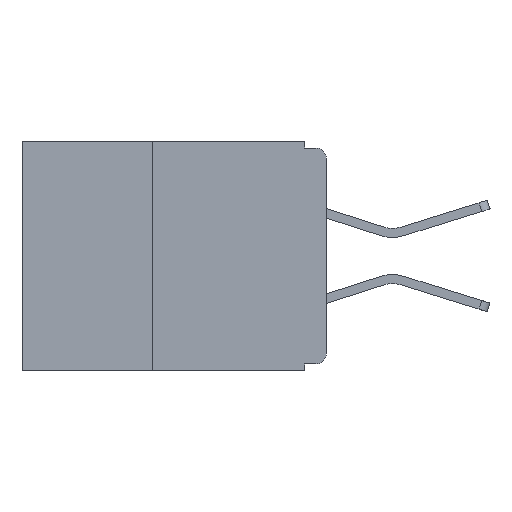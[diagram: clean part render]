
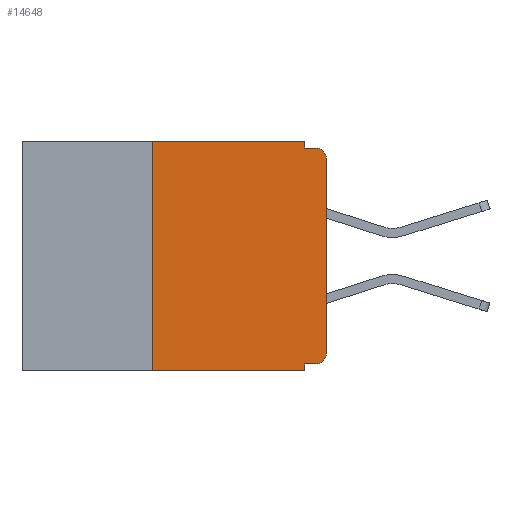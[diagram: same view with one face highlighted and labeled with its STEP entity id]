
A CAD part, left-side view. The second image highlights one B-rep face of the part: STEP entity #14648.
In plain terms, the highlighted planar face has unit normal (-1, 0, 0).
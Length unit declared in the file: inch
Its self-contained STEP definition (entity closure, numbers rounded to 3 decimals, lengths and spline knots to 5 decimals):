
#143 = LINE ( 'NONE', #12349, #18128 ) ;
#157 = VERTEX_POINT ( 'NONE', #21120 ) ;
#232 = DIRECTION ( 'NONE',  ( 0., 0., -1. ) ) ;
#410 = DIRECTION ( 'NONE',  ( 0., 0., -1. ) ) ;
#474 = DIRECTION ( 'NONE',  ( 0., -1., 0. ) ) ;
#589 = PLANE ( 'NONE',  #3066 ) ;
#1027 = LINE ( 'NONE', #11122, #20057 ) ;
#1802 = EDGE_CURVE ( 'NONE', #10880, #9495, #7541, .T. ) ;
#1854 = CARTESIAN_POINT ( 'NONE',  ( 0., 0.437, -0.33 ) ) ;
#2018 = VECTOR ( 'NONE', #2276, 39.37008 ) ;
#2039 = FACE_OUTER_BOUND ( 'NONE', #3339, .T. ) ;
#2276 = DIRECTION ( 'NONE',  ( 0., -1., 0. ) ) ;
#2361 = VECTOR ( 'NONE', #410, 39.37008 ) ;
#2442 = DIRECTION ( 'NONE',  ( 1., 0., 0. ) ) ;
#2985 = LINE ( 'NONE', #9601, #12583 ) ;
#3066 = AXIS2_PLACEMENT_3D ( 'NONE', #13242, #2442, #15018 ) ;
#3339 = EDGE_LOOP ( 'NONE', ( #22673, #15878, #10352, #20879, #21945, #16506, #5293, #3642, #5129, #12733 ) ) ;
#3525 = VECTOR ( 'NONE', #16379, 39.37008 ) ;
#3642 = ORIENTED_EDGE ( 'NONE', *, *, #8073, .F. ) ;
#4120 = CARTESIAN_POINT ( 'NONE',  ( 0., 0.437, 0. ) ) ;
#5129 = ORIENTED_EDGE ( 'NONE', *, *, #21127, .F. ) ;
#5293 = ORIENTED_EDGE ( 'NONE', *, *, #1802, .T. ) ;
#5303 = EDGE_CURVE ( 'NONE', #10880, #18103, #143, .T. ) ;
#6342 = CARTESIAN_POINT ( 'NONE',  ( 0., 0., 0. ) ) ;
#7115 = CARTESIAN_POINT ( 'NONE',  ( 0., 0.25, 0. ) ) ;
#7248 = AXIS2_PLACEMENT_3D ( 'NONE', #18072, #7424, #19826 ) ;
#7424 = DIRECTION ( 'NONE',  ( -1., 0., 0. ) ) ;
#7541 = LINE ( 'NONE', #1854, #11209 ) ;
#7942 = VERTEX_POINT ( 'NONE', #9191 ) ;
#8073 = EDGE_CURVE ( 'NONE', #7942, #9495, #21308, .T. ) ;
#9191 = CARTESIAN_POINT ( 'NONE',  ( 0., 0.031, -0.32 ) ) ;
#9495 = VERTEX_POINT ( 'NONE', #17965 ) ;
#9601 = CARTESIAN_POINT ( 'NONE',  ( 0., 0., -0.01 ) ) ;
#9658 = CARTESIAN_POINT ( 'NONE',  ( 0., 0.015, -0.01 ) ) ;
#9702 = CARTESIAN_POINT ( 'NONE',  ( 0., 0.015, -0.025 ) ) ;
#10116 = CIRCLE ( 'NONE', #7248, 0.015 ) ;
#10352 = ORIENTED_EDGE ( 'NONE', *, *, #22481, .F. ) ;
#10839 = EDGE_CURVE ( 'NONE', #19316, #157, #1027, .T. ) ;
#10851 = CARTESIAN_POINT ( 'NONE',  ( 0., 0.015, -0.32 ) ) ;
#10880 = VERTEX_POINT ( 'NONE', #14759 ) ;
#10893 = CARTESIAN_POINT ( 'NONE',  ( 0., 0., -0.305 ) ) ;
#11117 = EDGE_CURVE ( 'NONE', #19611, #15234, #19220, .T. ) ;
#11122 = CARTESIAN_POINT ( 'NONE',  ( 0., 0.031, 0. ) ) ;
#11209 = VECTOR ( 'NONE', #474, 39.37008 ) ;
#11284 = CARTESIAN_POINT ( 'NONE',  ( 0., 0.031, -0.33 ) ) ;
#11481 = DIRECTION ( 'NONE',  ( 0., 0., -1. ) ) ;
#12349 = CARTESIAN_POINT ( 'NONE',  ( 0., 0.25, -0.33 ) ) ;
#12418 = DIRECTION ( 'NONE',  ( 0., 0., 1. ) ) ;
#12583 = VECTOR ( 'NONE', #21886, 39.37008 ) ;
#12698 = VERTEX_POINT ( 'NONE', #10851 ) ;
#12733 = ORIENTED_EDGE ( 'NONE', *, *, #20473, .T. ) ;
#12752 = CARTESIAN_POINT ( 'NONE',  ( 0., 0., -0.32 ) ) ;
#13106 = LINE ( 'NONE', #12752, #3525 ) ;
#13242 = CARTESIAN_POINT ( 'NONE',  ( 0., 0.437, 0. ) ) ;
#13486 = DIRECTION ( 'NONE',  ( 0., 0., 1. ) ) ;
#14648 = ADVANCED_FACE ( 'NONE', ( #2039 ), #589, .F. ) ;
#14759 = CARTESIAN_POINT ( 'NONE',  ( 0., 0.25, -0.33 ) ) ;
#15018 = DIRECTION ( 'NONE',  ( 0., 0., -1. ) ) ;
#15234 = VERTEX_POINT ( 'NONE', #9658 ) ;
#15289 = CARTESIAN_POINT ( 'NONE',  ( 0., 0., -0.025 ) ) ;
#15878 = ORIENTED_EDGE ( 'NONE', *, *, #11117, .T. ) ;
#15984 = EDGE_CURVE ( 'NONE', #18647, #19611, #17479, .T. ) ;
#16379 = DIRECTION ( 'NONE',  ( 0., 1., 0. ) ) ;
#16453 = EDGE_CURVE ( 'NONE', #18103, #19316, #21000, .T. ) ;
#16506 = ORIENTED_EDGE ( 'NONE', *, *, #5303, .F. ) ;
#17479 = LINE ( 'NONE', #6342, #21561 ) ;
#17965 = CARTESIAN_POINT ( 'NONE',  ( 0., 0.031, -0.33 ) ) ;
#18072 = CARTESIAN_POINT ( 'NONE',  ( 0., 0.015, -0.305 ) ) ;
#18103 = VERTEX_POINT ( 'NONE', #7115 ) ;
#18128 = VECTOR ( 'NONE', #12418, 39.37008 ) ;
#18647 = VERTEX_POINT ( 'NONE', #10893 ) ;
#18841 = AXIS2_PLACEMENT_3D ( 'NONE', #9702, #21980, #11481 ) ;
#19220 = CIRCLE ( 'NONE', #18841, 0.015 ) ;
#19316 = VERTEX_POINT ( 'NONE', #19866 ) ;
#19611 = VERTEX_POINT ( 'NONE', #15289 ) ;
#19826 = DIRECTION ( 'NONE',  ( 0., 0., -1. ) ) ;
#19866 = CARTESIAN_POINT ( 'NONE',  ( 0., 0.031, 0. ) ) ;
#20057 = VECTOR ( 'NONE', #232, 39.37008 ) ;
#20473 = EDGE_CURVE ( 'NONE', #12698, #18647, #10116, .T. ) ;
#20879 = ORIENTED_EDGE ( 'NONE', *, *, #10839, .F. ) ;
#21000 = LINE ( 'NONE', #4120, #2018 ) ;
#21120 = CARTESIAN_POINT ( 'NONE',  ( 0., 0.031, -0.01 ) ) ;
#21127 = EDGE_CURVE ( 'NONE', #12698, #7942, #13106, .T. ) ;
#21308 = LINE ( 'NONE', #11284, #2361 ) ;
#21561 = VECTOR ( 'NONE', #13486, 39.37008 ) ;
#21886 = DIRECTION ( 'NONE',  ( 0., -1., 0. ) ) ;
#21945 = ORIENTED_EDGE ( 'NONE', *, *, #16453, .F. ) ;
#21980 = DIRECTION ( 'NONE',  ( -1., 0., 0. ) ) ;
#22481 = EDGE_CURVE ( 'NONE', #157, #15234, #2985, .T. ) ;
#22673 = ORIENTED_EDGE ( 'NONE', *, *, #15984, .T. ) ;
